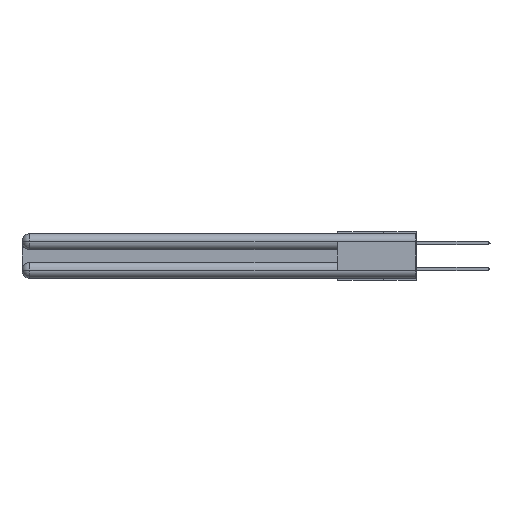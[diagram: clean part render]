
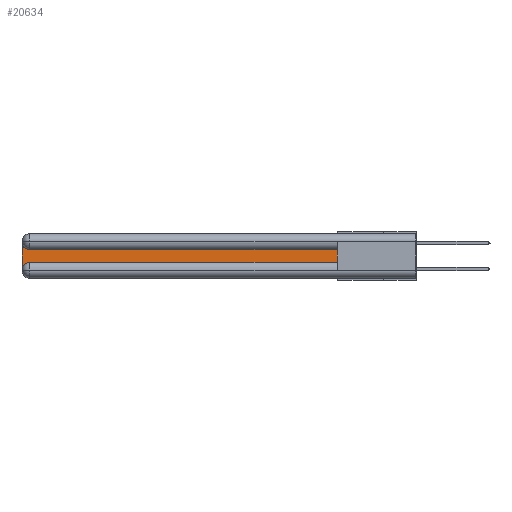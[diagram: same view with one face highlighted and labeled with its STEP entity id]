
A CAD part, left-side view. The second image highlights one B-rep face of the part: STEP entity #20634.
In plain terms, the highlighted planar face has unit normal (-1, 0, 0).
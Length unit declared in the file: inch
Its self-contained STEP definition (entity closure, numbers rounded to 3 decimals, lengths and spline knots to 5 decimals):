
#859 = CARTESIAN_POINT ( 'NONE',  ( 0.075, 3., -0.2775 ) ) ;
#1396 = EDGE_CURVE ( 'NONE', #28534, #20415, #26516, .T. ) ;
#1786 = DIRECTION ( 'NONE',  ( 1., 0., 0. ) ) ;
#2908 = AXIS2_PLACEMENT_3D ( 'NONE', #9031, #13292, #26364 ) ;
#2952 = AXIS2_PLACEMENT_3D ( 'NONE', #10477, #10773, #15234 ) ;
#2977 = CARTESIAN_POINT ( 'NONE',  ( 0.075, 2.94, -0.1225 ) ) ;
#3035 = ORIENTED_EDGE ( 'NONE', *, *, #6200, .T. ) ;
#3362 = CIRCLE ( 'NONE', #28478, 0.06 ) ;
#3384 = CARTESIAN_POINT ( 'NONE',  ( 0.075, 3., -0.2175 ) ) ;
#3809 = ORIENTED_EDGE ( 'NONE', *, *, #18869, .T. ) ;
#4105 = DIRECTION ( 'NONE',  ( 0., 1., 0. ) ) ;
#4278 = VECTOR ( 'NONE', #27791, 39.37008 ) ;
#5120 = VECTOR ( 'NONE', #4105, 39.37008 ) ;
#5782 = ORIENTED_EDGE ( 'NONE', *, *, #11275, .T. ) ;
#5910 = CARTESIAN_POINT ( 'NONE',  ( 0.075, 0.6, -0.2175 ) ) ;
#6156 = CARTESIAN_POINT ( 'NONE',  ( 0.075, 0.6, -0.1225 ) ) ;
#6200 = EDGE_CURVE ( 'NONE', #14902, #25735, #26320, .T. ) ;
#6540 = CARTESIAN_POINT ( 'NONE',  ( 0.075, 3., -0.0625 ) ) ;
#6832 = DIRECTION ( 'NONE',  ( 0., -1., 0. ) ) ;
#7414 = LINE ( 'NONE', #12175, #4278 ) ;
#8227 = EDGE_LOOP ( 'NONE', ( #3035, #13566, #3809, #5782, #21089, #14473 ) ) ;
#8876 = CARTESIAN_POINT ( 'NONE',  ( 0.075, 0.6, -0.2175 ) ) ;
#9031 = CARTESIAN_POINT ( 'NONE',  ( 0.075, 3., -0.1225 ) ) ;
#9476 = LINE ( 'NONE', #3384, #18806 ) ;
#10021 = DIRECTION ( 'NONE',  ( 0., 0., -1. ) ) ;
#10197 = VECTOR ( 'NONE', #6832, 39.37008 ) ;
#10477 = CARTESIAN_POINT ( 'NONE',  ( 0.075, 2.94, -0.2775 ) ) ;
#10773 = DIRECTION ( 'NONE',  ( 1., 0., 0. ) ) ;
#10869 = CARTESIAN_POINT ( 'NONE',  ( 0.075, 2.94, -0.0625 ) ) ;
#11070 = FACE_OUTER_BOUND ( 'NONE', #8227, .T. ) ;
#11275 = EDGE_CURVE ( 'NONE', #18031, #28534, #25326, .T. ) ;
#12175 = CARTESIAN_POINT ( 'NONE',  ( 0.075, 0.6, -0.2175 ) ) ;
#12324 = DIRECTION ( 'NONE',  ( 0., 0., -1. ) ) ;
#13292 = DIRECTION ( 'NONE',  ( 1., 0., 0. ) ) ;
#13566 = ORIENTED_EDGE ( 'NONE', *, *, #24937, .T. ) ;
#14429 = VERTEX_POINT ( 'NONE', #6540 ) ;
#14473 = ORIENTED_EDGE ( 'NONE', *, *, #23610, .T. ) ;
#14774 = CARTESIAN_POINT ( 'NONE',  ( 0.075, 2.94, -0.2175 ) ) ;
#14902 = VERTEX_POINT ( 'NONE', #18933 ) ;
#15234 = DIRECTION ( 'NONE',  ( 0., 0., -1. ) ) ;
#18031 = VERTEX_POINT ( 'NONE', #859 ) ;
#18806 = VECTOR ( 'NONE', #10021, 39.37008 ) ;
#18869 = EDGE_CURVE ( 'NONE', #14429, #18031, #9476, .T. ) ;
#18933 = CARTESIAN_POINT ( 'NONE',  ( 0.075, 0.6, -0.1225 ) ) ;
#20415 = VERTEX_POINT ( 'NONE', #5910 ) ;
#20634 = ADVANCED_FACE ( 'NONE', ( #11070 ), #26468, .F. ) ;
#21089 = ORIENTED_EDGE ( 'NONE', *, *, #1396, .T. ) ;
#23610 = EDGE_CURVE ( 'NONE', #20415, #14902, #7414, .T. ) ;
#24937 = EDGE_CURVE ( 'NONE', #25735, #14429, #3362, .T. ) ;
#25326 = CIRCLE ( 'NONE', #2952, 0.06 ) ;
#25735 = VERTEX_POINT ( 'NONE', #2977 ) ;
#26320 = LINE ( 'NONE', #6156, #5120 ) ;
#26364 = DIRECTION ( 'NONE',  ( 0., 0., -1. ) ) ;
#26468 = PLANE ( 'NONE',  #2908 ) ;
#26516 = LINE ( 'NONE', #8876, #10197 ) ;
#27791 = DIRECTION ( 'NONE',  ( 0., 0., 1. ) ) ;
#28478 = AXIS2_PLACEMENT_3D ( 'NONE', #10869, #1786, #12324 ) ;
#28534 = VERTEX_POINT ( 'NONE', #14774 ) ;
